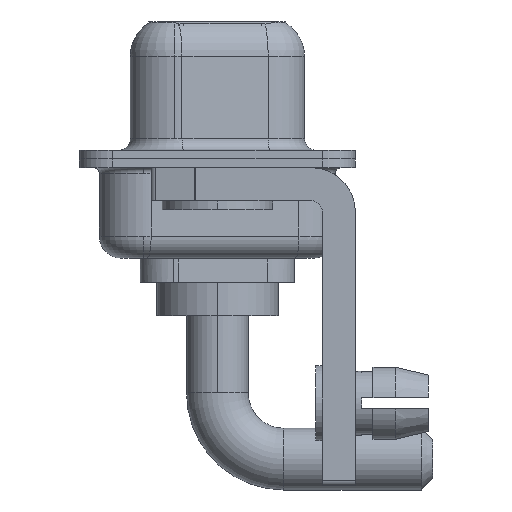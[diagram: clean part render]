
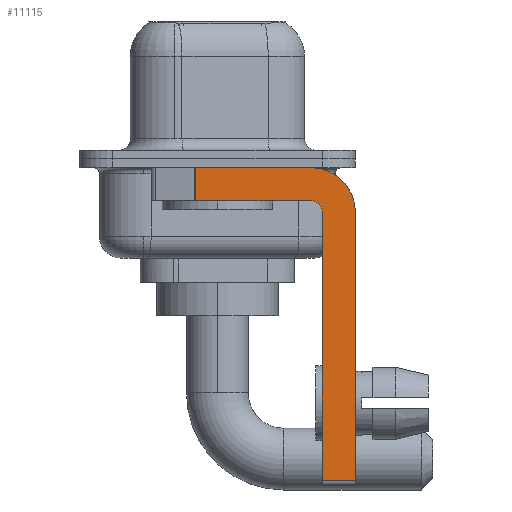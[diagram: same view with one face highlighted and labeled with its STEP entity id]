
A CAD part, left-side view. The second image highlights one B-rep face of the part: STEP entity #11115.
In plain terms, the highlighted planar face has unit normal (-1, 0, 0).
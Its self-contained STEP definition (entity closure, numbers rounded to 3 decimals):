
#198 = ORIENTED_EDGE ( 'NONE', *, *, #10369, .T. ) ;
#205 = CARTESIAN_POINT ( 'NONE',  ( -2.9, 0.978, -1.9 ) ) ;
#432 = EDGE_CURVE ( 'NONE', #6333, #1571, #14290, .T. ) ;
#547 = ORIENTED_EDGE ( 'NONE', *, *, #6465, .T. ) ;
#575 = VERTEX_POINT ( 'NONE', #10329 ) ;
#807 = CARTESIAN_POINT ( 'NONE',  ( -2.9, 3., -0.4 ) ) ;
#932 = CARTESIAN_POINT ( 'NONE',  ( -2.9, -4.25, -14.55 ) ) ;
#1264 = EDGE_CURVE ( 'NONE', #12858, #8480, #2299, .T. ) ;
#1544 = CARTESIAN_POINT ( 'NONE',  ( -2.9, -6.25, -2.4 ) ) ;
#1571 = VERTEX_POINT ( 'NONE', #205 ) ;
#1690 = LINE ( 'NONE', #3995, #11649 ) ;
#2035 = EDGE_CURVE ( 'NONE', #11216, #4312, #1690, .T. ) ;
#2109 = CARTESIAN_POINT ( 'NONE',  ( -2.9, 0.978, -1.9 ) ) ;
#2123 = VECTOR ( 'NONE', #7968, 1000. ) ;
#2125 = AXIS2_PLACEMENT_3D ( 'NONE', #2826, #7381, #11926 ) ;
#2147 = VECTOR ( 'NONE', #9893, 1000. ) ;
#2299 = LINE ( 'NONE', #13638, #2123 ) ;
#2338 = CARTESIAN_POINT ( 'NONE',  ( -2.9, -4.25, -1.9 ) ) ;
#2676 = DIRECTION ( 'NONE',  ( 0., 0., -1. ) ) ;
#2826 = CARTESIAN_POINT ( 'NONE',  ( -2.9, -4.25, -2.4 ) ) ;
#3995 = CARTESIAN_POINT ( 'NONE',  ( -2.9, -4.75, -14.8 ) ) ;
#4312 = VERTEX_POINT ( 'NONE', #8438 ) ;
#4381 = EDGE_CURVE ( 'NONE', #575, #12858, #6174, .T. ) ;
#4824 = FACE_OUTER_BOUND ( 'NONE', #12470, .T. ) ;
#5062 = EDGE_CURVE ( 'NONE', #4312, #6333, #13647, .T. ) ;
#6085 = CARTESIAN_POINT ( 'NONE',  ( -2.9, 0.978, -0.4 ) ) ;
#6174 = CIRCLE ( 'NONE', #2125, 2. ) ;
#6283 = AXIS2_PLACEMENT_3D ( 'NONE', #12819, #11701, #2676 ) ;
#6333 = VERTEX_POINT ( 'NONE', #2338 ) ;
#6465 = EDGE_CURVE ( 'NONE', #11216, #8480, #13752, .T. ) ;
#6964 = ORIENTED_EDGE ( 'NONE', *, *, #432, .F. ) ;
#7381 = DIRECTION ( 'NONE',  ( 1., 0., 0. ) ) ;
#7582 = DIRECTION ( 'NONE',  ( 0., 1., 0. ) ) ;
#7651 = CARTESIAN_POINT ( 'NONE',  ( -2.9, -4.25, -1.9 ) ) ;
#7832 = ORIENTED_EDGE ( 'NONE', *, *, #4381, .F. ) ;
#7968 = DIRECTION ( 'NONE',  ( 0., 0., -1. ) ) ;
#8332 = DIRECTION ( 'NONE',  ( 0., 0., 1. ) ) ;
#8438 = CARTESIAN_POINT ( 'NONE',  ( -2.9, -4.75, -2.4 ) ) ;
#8469 = EDGE_CURVE ( 'NONE', #9707, #575, #9822, .T. ) ;
#8472 = CARTESIAN_POINT ( 'NONE',  ( -2.9, -4.25, -2.4 ) ) ;
#8480 = VERTEX_POINT ( 'NONE', #14364 ) ;
#9055 = LINE ( 'NONE', #2109, #11478 ) ;
#9663 = DIRECTION ( 'NONE',  ( 0., 0., 1. ) ) ;
#9707 = VERTEX_POINT ( 'NONE', #6085 ) ;
#9822 = LINE ( 'NONE', #807, #2147 ) ;
#9893 = DIRECTION ( 'NONE',  ( 0., -1., 0. ) ) ;
#10158 = ORIENTED_EDGE ( 'NONE', *, *, #5062, .F. ) ;
#10241 = DIRECTION ( 'NONE',  ( 0., -1., 0. ) ) ;
#10329 = CARTESIAN_POINT ( 'NONE',  ( -2.9, -4.25, -0.4 ) ) ;
#10369 = EDGE_CURVE ( 'NONE', #9707, #1571, #9055, .T. ) ;
#10605 = ORIENTED_EDGE ( 'NONE', *, *, #2035, .F. ) ;
#10772 = DIRECTION ( 'NONE',  ( -1., 0., 0. ) ) ;
#11115 = ADVANCED_FACE ( 'NONE', ( #4824 ), #12971, .F. ) ;
#11216 = VERTEX_POINT ( 'NONE', #12141 ) ;
#11253 = AXIS2_PLACEMENT_3D ( 'NONE', #8472, #10772, #9663 ) ;
#11478 = VECTOR ( 'NONE', #14500, 1000. ) ;
#11483 = VECTOR ( 'NONE', #7582, 1000. ) ;
#11649 = VECTOR ( 'NONE', #8332, 1000. ) ;
#11701 = DIRECTION ( 'NONE',  ( 1., 0., 0. ) ) ;
#11926 = DIRECTION ( 'NONE',  ( 0., 0., -1. ) ) ;
#12141 = CARTESIAN_POINT ( 'NONE',  ( -2.9, -4.75, -14.55 ) ) ;
#12470 = EDGE_LOOP ( 'NONE', ( #13098, #198, #6964, #10158, #10605, #547, #13668, #7832 ) ) ;
#12819 = CARTESIAN_POINT ( 'NONE',  ( -2.9, -4.25, -2.4 ) ) ;
#12858 = VERTEX_POINT ( 'NONE', #1544 ) ;
#12971 = PLANE ( 'NONE',  #6283 ) ;
#13098 = ORIENTED_EDGE ( 'NONE', *, *, #8469, .F. ) ;
#13375 = VECTOR ( 'NONE', #10241, 1000. ) ;
#13638 = CARTESIAN_POINT ( 'NONE',  ( -2.9, -6.25, -2.4 ) ) ;
#13647 = CIRCLE ( 'NONE', #11253, 0.5 ) ;
#13668 = ORIENTED_EDGE ( 'NONE', *, *, #1264, .F. ) ;
#13752 = LINE ( 'NONE', #932, #13375 ) ;
#14290 = LINE ( 'NONE', #7651, #11483 ) ;
#14364 = CARTESIAN_POINT ( 'NONE',  ( -2.9, -6.25, -14.55 ) ) ;
#14500 = DIRECTION ( 'NONE',  ( 0., 0., -1. ) ) ;
